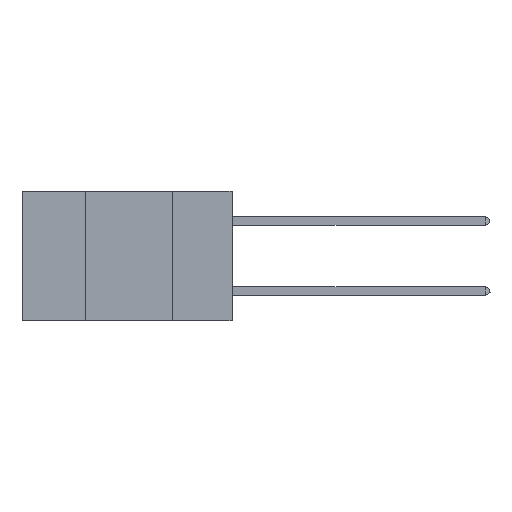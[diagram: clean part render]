
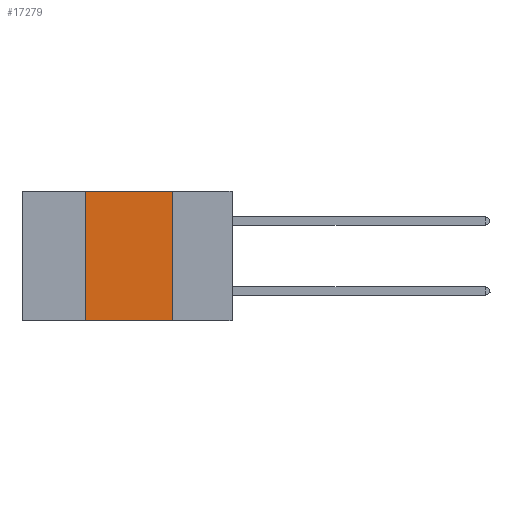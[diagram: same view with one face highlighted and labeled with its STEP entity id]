
A CAD part, left-side view. The second image highlights one B-rep face of the part: STEP entity #17279.
In plain terms, the highlighted planar face has unit normal (-1, 0, 0).
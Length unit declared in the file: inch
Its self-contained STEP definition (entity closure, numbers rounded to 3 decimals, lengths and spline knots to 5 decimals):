
#866 = EDGE_LOOP ( 'NONE', ( #6309, #5923, #26039, #4730 ) ) ;
#2597 = LINE ( 'NONE', #30856, #30884 ) ;
#3267 = VERTEX_POINT ( 'NONE', #31429 ) ;
#4730 = ORIENTED_EDGE ( 'NONE', *, *, #25801, .T. ) ;
#5923 = ORIENTED_EDGE ( 'NONE', *, *, #26002, .F. ) ;
#6137 = AXIS2_PLACEMENT_3D ( 'NONE', #25509, #6684, #17380 ) ;
#6309 = ORIENTED_EDGE ( 'NONE', *, *, #19236, .F. ) ;
#6311 = PLANE ( 'NONE',  #6137 ) ;
#6684 = DIRECTION ( 'NONE',  ( 1., 0., 0. ) ) ;
#7145 = CARTESIAN_POINT ( 'NONE',  ( 0., 0.17, 0. ) ) ;
#7163 = VERTEX_POINT ( 'NONE', #21050 ) ;
#7667 = CARTESIAN_POINT ( 'NONE',  ( 0., 0.42, -0.37 ) ) ;
#10737 = FACE_OUTER_BOUND ( 'NONE', #866, .T. ) ;
#13116 = CARTESIAN_POINT ( 'NONE',  ( 0., 0.42, 0. ) ) ;
#13242 = VERTEX_POINT ( 'NONE', #7667 ) ;
#14732 = VECTOR ( 'NONE', #35447, 39.37008 ) ;
#17279 = ADVANCED_FACE ( 'NONE', ( #10737 ), #6311, .F. ) ;
#17380 = DIRECTION ( 'NONE',  ( 0., 0., -1. ) ) ;
#18910 = CARTESIAN_POINT ( 'NONE',  ( 0., 0.42, 0. ) ) ;
#19236 = EDGE_CURVE ( 'NONE', #3267, #7163, #21799, .T. ) ;
#21050 = CARTESIAN_POINT ( 'NONE',  ( 0., 0.17, -0.37 ) ) ;
#21553 = DIRECTION ( 'NONE',  ( 0., -1., 0. ) ) ;
#21784 = CARTESIAN_POINT ( 'NONE',  ( 0., 0.6, -0.37 ) ) ;
#21799 = LINE ( 'NONE', #7145, #29945 ) ;
#23253 = EDGE_CURVE ( 'NONE', #13242, #25709, #27250, .T. ) ;
#25509 = CARTESIAN_POINT ( 'NONE',  ( 0., 0.6, 0. ) ) ;
#25709 = VERTEX_POINT ( 'NONE', #18910 ) ;
#25801 = EDGE_CURVE ( 'NONE', #13242, #7163, #33504, .T. ) ;
#26002 = EDGE_CURVE ( 'NONE', #25709, #3267, #2597, .T. ) ;
#26039 = ORIENTED_EDGE ( 'NONE', *, *, #23253, .F. ) ;
#26321 = DIRECTION ( 'NONE',  ( 0., 0., -1. ) ) ;
#27250 = LINE ( 'NONE', #13116, #14732 ) ;
#27937 = VECTOR ( 'NONE', #21553, 39.37008 ) ;
#29945 = VECTOR ( 'NONE', #26321, 39.37008 ) ;
#30856 = CARTESIAN_POINT ( 'NONE',  ( 0., 0.6, 0. ) ) ;
#30884 = VECTOR ( 'NONE', #33902, 39.37008 ) ;
#31429 = CARTESIAN_POINT ( 'NONE',  ( 0., 0.17, 0. ) ) ;
#33504 = LINE ( 'NONE', #21784, #27937 ) ;
#33902 = DIRECTION ( 'NONE',  ( 0., -1., 0. ) ) ;
#35447 = DIRECTION ( 'NONE',  ( 0., 0., 1. ) ) ;
